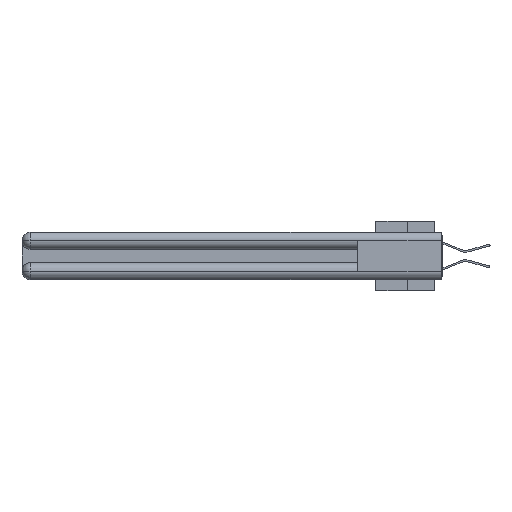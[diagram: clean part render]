
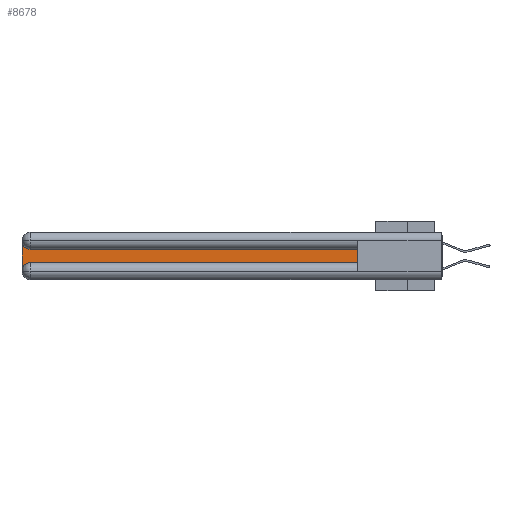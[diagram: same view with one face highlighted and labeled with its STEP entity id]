
A CAD part, left-side view. The second image highlights one B-rep face of the part: STEP entity #8678.
In plain terms, the highlighted planar face has unit normal (-1, 0, 0).
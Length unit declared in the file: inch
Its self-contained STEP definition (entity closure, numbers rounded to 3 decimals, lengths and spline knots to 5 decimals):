
#24 = VERTEX_POINT ( 'NONE', #37406 ) ;
#123 = VECTOR ( 'NONE', #6248, 39.37008 ) ;
#769 = ORIENTED_EDGE ( 'NONE', *, *, #14845, .T. ) ;
#2062 = ORIENTED_EDGE ( 'NONE', *, *, #35565, .T. ) ;
#2082 = CARTESIAN_POINT ( 'NONE',  ( 0.075, 0.6, -0.1225 ) ) ;
#3796 = LINE ( 'NONE', #2082, #16813 ) ;
#3944 = EDGE_CURVE ( 'NONE', #13486, #24, #17587, .T. ) ;
#5161 = DIRECTION ( 'NONE',  ( 0., 1., 0. ) ) ;
#5303 = VERTEX_POINT ( 'NONE', #12949 ) ;
#5571 = DIRECTION ( 'NONE',  ( 0., 0., -1. ) ) ;
#5611 = DIRECTION ( 'NONE',  ( 0., 0., -1. ) ) ;
#5755 = DIRECTION ( 'NONE',  ( 1., 0., 0. ) ) ;
#5906 = CARTESIAN_POINT ( 'NONE',  ( 0.075, 2.94, -0.2175 ) ) ;
#6248 = DIRECTION ( 'NONE',  ( 0., 0., -1. ) ) ;
#6638 = LINE ( 'NONE', #12965, #123 ) ;
#8250 = CARTESIAN_POINT ( 'NONE',  ( 0.075, 0.6, -0.1225 ) ) ;
#8678 = ADVANCED_FACE ( 'NONE', ( #37818 ), #21767, .F. ) ;
#8869 = LINE ( 'NONE', #18063, #26397 ) ;
#10956 = EDGE_LOOP ( 'NONE', ( #39072, #2062, #19039, #769, #26180, #32679 ) ) ;
#11830 = DIRECTION ( 'NONE',  ( 0., -1., 0. ) ) ;
#12949 = CARTESIAN_POINT ( 'NONE',  ( 0.075, 3., -0.2775 ) ) ;
#12965 = CARTESIAN_POINT ( 'NONE',  ( 0.075, 3., -0.2175 ) ) ;
#12998 = AXIS2_PLACEMENT_3D ( 'NONE', #21572, #18740, #5571 ) ;
#13486 = VERTEX_POINT ( 'NONE', #5906 ) ;
#13764 = EDGE_CURVE ( 'NONE', #24, #26623, #8869, .T. ) ;
#14805 = CIRCLE ( 'NONE', #26678, 0.06 ) ;
#14845 = EDGE_CURVE ( 'NONE', #5303, #13486, #14805, .T. ) ;
#16813 = VECTOR ( 'NONE', #5161, 39.37008 ) ;
#17587 = LINE ( 'NONE', #33880, #29611 ) ;
#18063 = CARTESIAN_POINT ( 'NONE',  ( 0.075, 0.6, -0.2175 ) ) ;
#18740 = DIRECTION ( 'NONE',  ( 1., 0., 0. ) ) ;
#19039 = ORIENTED_EDGE ( 'NONE', *, *, #36874, .T. ) ;
#20772 = CARTESIAN_POINT ( 'NONE',  ( 0.075, 3., -0.0625 ) ) ;
#21572 = CARTESIAN_POINT ( 'NONE',  ( 0.075, 2.94, -0.0625 ) ) ;
#21767 = PLANE ( 'NONE',  #36474 ) ;
#21905 = CARTESIAN_POINT ( 'NONE',  ( 0.075, 3., -0.1225 ) ) ;
#22362 = CIRCLE ( 'NONE', #12998, 0.06 ) ;
#24966 = DIRECTION ( 'NONE',  ( 1., 0., 0. ) ) ;
#26180 = ORIENTED_EDGE ( 'NONE', *, *, #3944, .T. ) ;
#26397 = VECTOR ( 'NONE', #33676, 39.37008 ) ;
#26623 = VERTEX_POINT ( 'NONE', #8250 ) ;
#26678 = AXIS2_PLACEMENT_3D ( 'NONE', #34683, #5755, #34550 ) ;
#27803 = CARTESIAN_POINT ( 'NONE',  ( 0.075, 2.94, -0.1225 ) ) ;
#29611 = VECTOR ( 'NONE', #11830, 39.37008 ) ;
#32679 = ORIENTED_EDGE ( 'NONE', *, *, #13764, .T. ) ;
#33589 = VERTEX_POINT ( 'NONE', #20772 ) ;
#33676 = DIRECTION ( 'NONE',  ( 0., 0., 1. ) ) ;
#33880 = CARTESIAN_POINT ( 'NONE',  ( 0.075, 0.6, -0.2175 ) ) ;
#34550 = DIRECTION ( 'NONE',  ( 0., 0., -1. ) ) ;
#34683 = CARTESIAN_POINT ( 'NONE',  ( 0.075, 2.94, -0.2775 ) ) ;
#35504 = EDGE_CURVE ( 'NONE', #26623, #37778, #3796, .T. ) ;
#35565 = EDGE_CURVE ( 'NONE', #37778, #33589, #22362, .T. ) ;
#36474 = AXIS2_PLACEMENT_3D ( 'NONE', #21905, #24966, #5611 ) ;
#36874 = EDGE_CURVE ( 'NONE', #33589, #5303, #6638, .T. ) ;
#37406 = CARTESIAN_POINT ( 'NONE',  ( 0.075, 0.6, -0.2175 ) ) ;
#37778 = VERTEX_POINT ( 'NONE', #27803 ) ;
#37818 = FACE_OUTER_BOUND ( 'NONE', #10956, .T. ) ;
#39072 = ORIENTED_EDGE ( 'NONE', *, *, #35504, .T. ) ;
